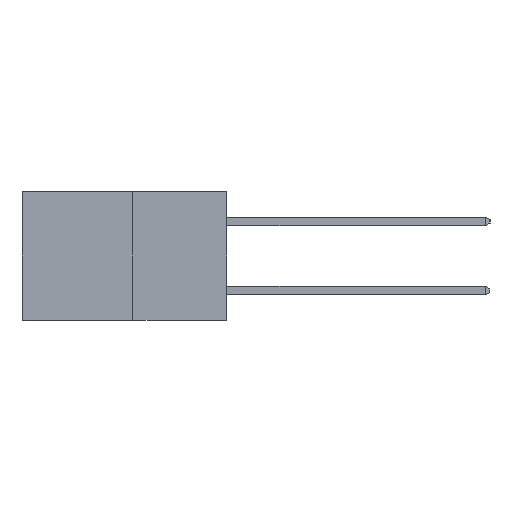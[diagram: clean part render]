
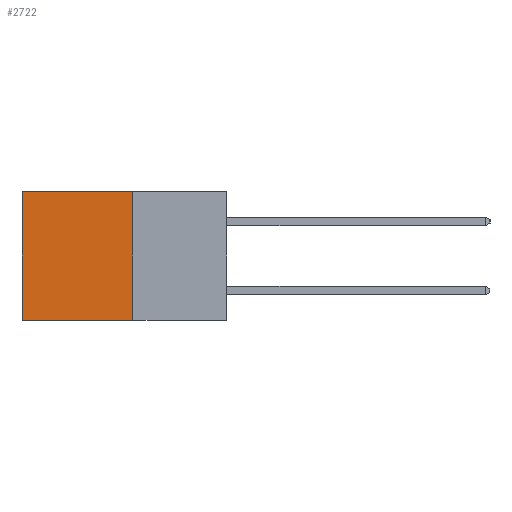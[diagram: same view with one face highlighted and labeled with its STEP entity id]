
A CAD part, left-side view. The second image highlights one B-rep face of the part: STEP entity #2722.
In plain terms, the highlighted planar face has unit normal (-1, 0, 0).
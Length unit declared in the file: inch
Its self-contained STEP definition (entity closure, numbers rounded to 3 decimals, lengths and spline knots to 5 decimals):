
#90 = CARTESIAN_POINT ( 'NONE',  ( 0.277, 0.27, 0. ) ) ;
#422 = CARTESIAN_POINT ( 'NONE',  ( 0.277, 0.59, -0.37 ) ) ;
#474 = EDGE_CURVE ( 'NONE', #5953, #13340, #4990, .T. ) ;
#1159 = PLANE ( 'NONE',  #8364 ) ;
#1380 = LINE ( 'NONE', #3671, #9306 ) ;
#1524 = EDGE_CURVE ( 'NONE', #8144, #8540, #1380, .T. ) ;
#1816 = DIRECTION ( 'NONE',  ( 1., 0., 0. ) ) ;
#2069 = DIRECTION ( 'NONE',  ( 0., 1., 0. ) ) ;
#2507 = CARTESIAN_POINT ( 'NONE',  ( 0.277, 0.59, -0.37 ) ) ;
#2636 = CARTESIAN_POINT ( 'NONE',  ( 0.277, 0.27, 0. ) ) ;
#2715 = DIRECTION ( 'NONE',  ( 0., 0., -1. ) ) ;
#2722 = ADVANCED_FACE ( 'NONE', ( #5584 ), #1159, .F. ) ;
#2852 = DIRECTION ( 'NONE',  ( 0., 0., -1. ) ) ;
#3671 = CARTESIAN_POINT ( 'NONE',  ( 0.277, 0.27, -0.37 ) ) ;
#4151 = ORIENTED_EDGE ( 'NONE', *, *, #1524, .F. ) ;
#4243 = LINE ( 'NONE', #2636, #6940 ) ;
#4990 = LINE ( 'NONE', #2507, #5316 ) ;
#5115 = ORIENTED_EDGE ( 'NONE', *, *, #5142, .T. ) ;
#5142 = EDGE_CURVE ( 'NONE', #8144, #5953, #4243, .T. ) ;
#5316 = VECTOR ( 'NONE', #2715, 39.37008 ) ;
#5398 = DIRECTION ( 'NONE',  ( 0., 1., 0. ) ) ;
#5584 = FACE_OUTER_BOUND ( 'NONE', #7918, .T. ) ;
#5953 = VERTEX_POINT ( 'NONE', #12659 ) ;
#6001 = CARTESIAN_POINT ( 'NONE',  ( 0.277, 0.27, -0.37 ) ) ;
#6940 = VECTOR ( 'NONE', #2069, 39.37008 ) ;
#7259 = CARTESIAN_POINT ( 'NONE',  ( 0.277, 0.27, -0.37 ) ) ;
#7385 = CARTESIAN_POINT ( 'NONE',  ( 0.277, 0.27, -0.37 ) ) ;
#7526 = VECTOR ( 'NONE', #5398, 39.37008 ) ;
#7918 = EDGE_LOOP ( 'NONE', ( #10408, #12809, #4151, #5115 ) ) ;
#8144 = VERTEX_POINT ( 'NONE', #90 ) ;
#8364 = AXIS2_PLACEMENT_3D ( 'NONE', #7259, #1816, #2852 ) ;
#8540 = VERTEX_POINT ( 'NONE', #6001 ) ;
#9306 = VECTOR ( 'NONE', #10018, 39.37008 ) ;
#10018 = DIRECTION ( 'NONE',  ( 0., 0., -1. ) ) ;
#10294 = LINE ( 'NONE', #7385, #7526 ) ;
#10408 = ORIENTED_EDGE ( 'NONE', *, *, #474, .T. ) ;
#11268 = EDGE_CURVE ( 'NONE', #8540, #13340, #10294, .T. ) ;
#12659 = CARTESIAN_POINT ( 'NONE',  ( 0.277, 0.59, 0. ) ) ;
#12809 = ORIENTED_EDGE ( 'NONE', *, *, #11268, .F. ) ;
#13340 = VERTEX_POINT ( 'NONE', #422 ) ;
